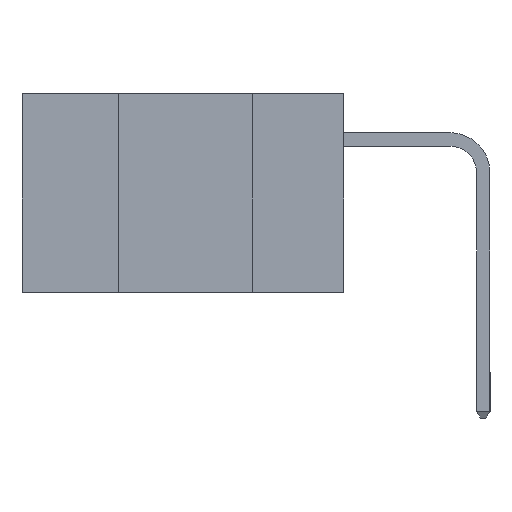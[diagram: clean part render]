
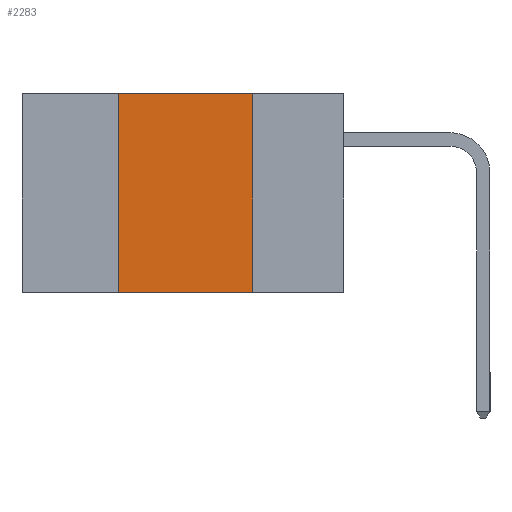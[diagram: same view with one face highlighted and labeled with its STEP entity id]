
A CAD part, left-side view. The second image highlights one B-rep face of the part: STEP entity #2283.
In plain terms, the highlighted planar face has unit normal (-1, 0, 0).
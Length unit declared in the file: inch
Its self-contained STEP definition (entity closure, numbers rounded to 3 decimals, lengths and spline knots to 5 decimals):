
#303 = VERTEX_POINT ( 'NONE', #6862 ) ;
#411 = AXIS2_PLACEMENT_3D ( 'NONE', #654, #6439, #4410 ) ;
#635 = CARTESIAN_POINT ( 'NONE',  ( 0., 0.17, 0. ) ) ;
#643 = EDGE_CURVE ( 'NONE', #7004, #3119, #5287, .T. ) ;
#654 = CARTESIAN_POINT ( 'NONE',  ( 0., 0.6, 0. ) ) ;
#752 = ORIENTED_EDGE ( 'NONE', *, *, #8106, .F. ) ;
#1118 = DIRECTION ( 'NONE',  ( 0., 0., 1. ) ) ;
#1291 = VECTOR ( 'NONE', #5712, 39.37008 ) ;
#1379 = VECTOR ( 'NONE', #1118, 39.37008 ) ;
#1920 = DIRECTION ( 'NONE',  ( 0., -1., 0. ) ) ;
#1933 = EDGE_LOOP ( 'NONE', ( #6520, #752, #2017, #8317 ) ) ;
#2017 = ORIENTED_EDGE ( 'NONE', *, *, #3811, .F. ) ;
#2283 = ADVANCED_FACE ( 'NONE', ( #7303 ), #8601, .F. ) ;
#2663 = VECTOR ( 'NONE', #1920, 39.37008 ) ;
#2854 = CARTESIAN_POINT ( 'NONE',  ( 0., 0.6, -0.37 ) ) ;
#3031 = VERTEX_POINT ( 'NONE', #8178 ) ;
#3119 = VERTEX_POINT ( 'NONE', #6698 ) ;
#3301 = CARTESIAN_POINT ( 'NONE',  ( 0., 0.42, 0. ) ) ;
#3628 = CARTESIAN_POINT ( 'NONE',  ( 0., 0.42, -0.37 ) ) ;
#3811 = EDGE_CURVE ( 'NONE', #7004, #3031, #4211, .T. ) ;
#4211 = LINE ( 'NONE', #3301, #1379 ) ;
#4410 = DIRECTION ( 'NONE',  ( 0., 0., -1. ) ) ;
#5287 = LINE ( 'NONE', #2854, #7099 ) ;
#5405 = DIRECTION ( 'NONE',  ( 0., -1., 0. ) ) ;
#5712 = DIRECTION ( 'NONE',  ( 0., 0., -1. ) ) ;
#5828 = LINE ( 'NONE', #635, #1291 ) ;
#6439 = DIRECTION ( 'NONE',  ( 1., 0., 0. ) ) ;
#6520 = ORIENTED_EDGE ( 'NONE', *, *, #7746, .F. ) ;
#6698 = CARTESIAN_POINT ( 'NONE',  ( 0., 0.17, -0.37 ) ) ;
#6737 = LINE ( 'NONE', #7691, #2663 ) ;
#6862 = CARTESIAN_POINT ( 'NONE',  ( 0., 0.17, 0. ) ) ;
#7004 = VERTEX_POINT ( 'NONE', #3628 ) ;
#7099 = VECTOR ( 'NONE', #5405, 39.37008 ) ;
#7303 = FACE_OUTER_BOUND ( 'NONE', #1933, .T. ) ;
#7691 = CARTESIAN_POINT ( 'NONE',  ( 0., 0.6, 0. ) ) ;
#7746 = EDGE_CURVE ( 'NONE', #303, #3119, #5828, .T. ) ;
#8106 = EDGE_CURVE ( 'NONE', #3031, #303, #6737, .T. ) ;
#8178 = CARTESIAN_POINT ( 'NONE',  ( 0., 0.42, 0. ) ) ;
#8317 = ORIENTED_EDGE ( 'NONE', *, *, #643, .T. ) ;
#8601 = PLANE ( 'NONE',  #411 ) ;
